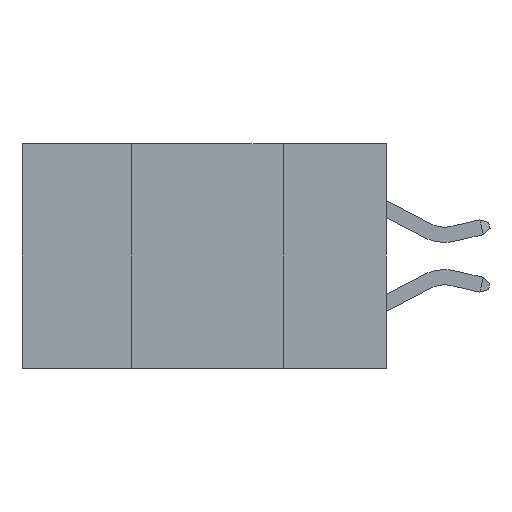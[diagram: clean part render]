
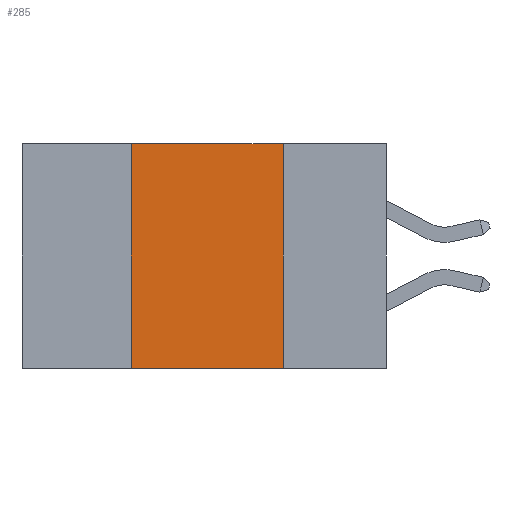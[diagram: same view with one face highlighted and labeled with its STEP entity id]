
A CAD part, left-side view. The second image highlights one B-rep face of the part: STEP entity #285.
In plain terms, the highlighted planar face has unit normal (-1, 0, 0).
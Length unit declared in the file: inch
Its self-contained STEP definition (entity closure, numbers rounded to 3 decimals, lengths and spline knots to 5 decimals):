
#285 = ADVANCED_FACE ( 'NONE', ( #15665 ), #18312, .F. ) ;
#335 = VECTOR ( 'NONE', #4132, 39.37008 ) ;
#530 = VECTOR ( 'NONE', #16462, 39.37008 ) ;
#770 = CARTESIAN_POINT ( 'NONE',  ( 0., 0.17, 0. ) ) ;
#1144 = CARTESIAN_POINT ( 'NONE',  ( 0., 0.17, -0.37 ) ) ;
#1456 = DIRECTION ( 'NONE',  ( 1., 0., 0. ) ) ;
#2175 = EDGE_LOOP ( 'NONE', ( #7489, #15984, #14218, #9677 ) ) ;
#2773 = CARTESIAN_POINT ( 'NONE',  ( 0., 0.42, 0. ) ) ;
#2818 = EDGE_CURVE ( 'NONE', #8996, #8268, #16379, .T. ) ;
#4132 = DIRECTION ( 'NONE',  ( 0., -1., 0. ) ) ;
#4402 = VECTOR ( 'NONE', #19686, 39.37008 ) ;
#5527 = LINE ( 'NONE', #22984, #335 ) ;
#7489 = ORIENTED_EDGE ( 'NONE', *, *, #16403, .F. ) ;
#7627 = LINE ( 'NONE', #770, #4402 ) ;
#7750 = CARTESIAN_POINT ( 'NONE',  ( 0., 0.17, 0. ) ) ;
#8268 = VERTEX_POINT ( 'NONE', #21453 ) ;
#8342 = AXIS2_PLACEMENT_3D ( 'NONE', #12526, #1456, #14452 ) ;
#8996 = VERTEX_POINT ( 'NONE', #21889 ) ;
#9677 = ORIENTED_EDGE ( 'NONE', *, *, #10679, .T. ) ;
#10679 = EDGE_CURVE ( 'NONE', #8996, #11701, #19059, .T. ) ;
#11617 = VECTOR ( 'NONE', #15687, 39.37008 ) ;
#11701 = VERTEX_POINT ( 'NONE', #1144 ) ;
#12526 = CARTESIAN_POINT ( 'NONE',  ( 0., 0.6, 0. ) ) ;
#14218 = ORIENTED_EDGE ( 'NONE', *, *, #2818, .F. ) ;
#14452 = DIRECTION ( 'NONE',  ( 0., 0., -1. ) ) ;
#15609 = CARTESIAN_POINT ( 'NONE',  ( 0., 0.6, -0.37 ) ) ;
#15665 = FACE_OUTER_BOUND ( 'NONE', #2175, .T. ) ;
#15687 = DIRECTION ( 'NONE',  ( 0., -1., 0. ) ) ;
#15984 = ORIENTED_EDGE ( 'NONE', *, *, #18025, .F. ) ;
#16173 = VERTEX_POINT ( 'NONE', #7750 ) ;
#16379 = LINE ( 'NONE', #2773, #530 ) ;
#16403 = EDGE_CURVE ( 'NONE', #16173, #11701, #7627, .T. ) ;
#16462 = DIRECTION ( 'NONE',  ( 0., 0., 1. ) ) ;
#18025 = EDGE_CURVE ( 'NONE', #8268, #16173, #5527, .T. ) ;
#18312 = PLANE ( 'NONE',  #8342 ) ;
#19059 = LINE ( 'NONE', #15609, #11617 ) ;
#19686 = DIRECTION ( 'NONE',  ( 0., 0., -1. ) ) ;
#21453 = CARTESIAN_POINT ( 'NONE',  ( 0., 0.42, 0. ) ) ;
#21889 = CARTESIAN_POINT ( 'NONE',  ( 0., 0.42, -0.37 ) ) ;
#22984 = CARTESIAN_POINT ( 'NONE',  ( 0., 0.6, 0. ) ) ;
